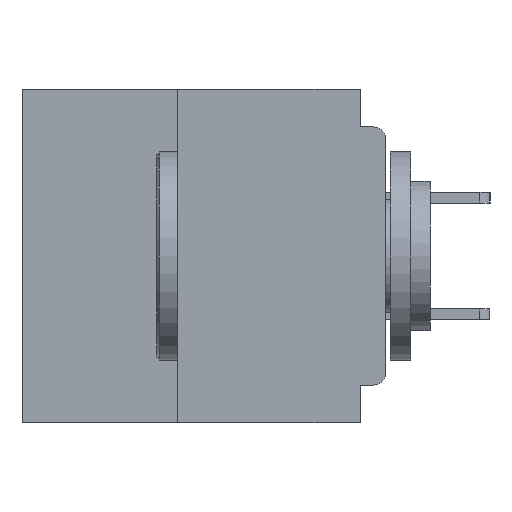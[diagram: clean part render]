
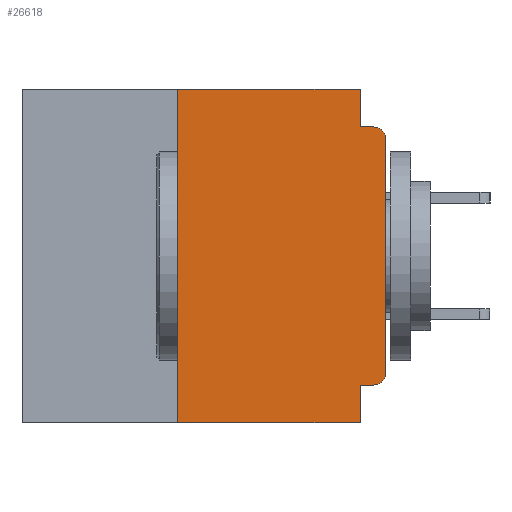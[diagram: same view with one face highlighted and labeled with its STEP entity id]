
A CAD part, left-side view. The second image highlights one B-rep face of the part: STEP entity #26618.
In plain terms, the highlighted planar face has unit normal (-1, 0, 0).
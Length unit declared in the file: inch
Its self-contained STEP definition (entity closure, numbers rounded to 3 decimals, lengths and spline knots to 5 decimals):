
#1320 = EDGE_CURVE ( 'NONE', #28242, #49609, #9044, .T. ) ;
#1909 = VERTEX_POINT ( 'NONE', #51159 ) ;
#2631 = DIRECTION ( 'NONE',  ( 0., 0., -1. ) ) ;
#3172 = ORIENTED_EDGE ( 'NONE', *, *, #53670, .T. ) ;
#4496 = DIRECTION ( 'NONE',  ( 0., 0., -1. ) ) ;
#6060 = VERTEX_POINT ( 'NONE', #48987 ) ;
#6602 = AXIS2_PLACEMENT_3D ( 'NONE', #45003, #19979, #49123 ) ;
#7800 = ORIENTED_EDGE ( 'NONE', *, *, #20304, .T. ) ;
#7839 = VECTOR ( 'NONE', #15477, 39.37008 ) ;
#7906 = LINE ( 'NONE', #22222, #30171 ) ;
#8903 = CARTESIAN_POINT ( 'NONE',  ( 0., 0.031, 0. ) ) ;
#9044 = LINE ( 'NONE', #44991, #41119 ) ;
#9107 = CARTESIAN_POINT ( 'NONE',  ( 0., 0., 0. ) ) ;
#10751 = LINE ( 'NONE', #48096, #52468 ) ;
#11008 = VECTOR ( 'NONE', #21540, 39.37008 ) ;
#12339 = CARTESIAN_POINT ( 'NONE',  ( 0., 0.437, -0.4 ) ) ;
#12829 = ORIENTED_EDGE ( 'NONE', *, *, #1320, .F. ) ;
#13657 = LINE ( 'NONE', #50643, #11008 ) ;
#14400 = ORIENTED_EDGE ( 'NONE', *, *, #47520, .T. ) ;
#15447 = VERTEX_POINT ( 'NONE', #40591 ) ;
#15477 = DIRECTION ( 'NONE',  ( 0., 0., 1. ) ) ;
#15708 = EDGE_CURVE ( 'NONE', #39594, #44630, #27010, .T. ) ;
#17530 = DIRECTION ( 'NONE',  ( 0., 0., 1. ) ) ;
#19979 = DIRECTION ( 'NONE',  ( -1., 0., 0. ) ) ;
#20304 = EDGE_CURVE ( 'NONE', #48693, #1909, #52551, .T. ) ;
#20799 = CIRCLE ( 'NONE', #35725, 0.015 ) ;
#21540 = DIRECTION ( 'NONE',  ( 0., -1., 0. ) ) ;
#21564 = LINE ( 'NONE', #9107, #42482 ) ;
#22110 = CARTESIAN_POINT ( 'NONE',  ( 0., 0.015, -0.355 ) ) ;
#22222 = CARTESIAN_POINT ( 'NONE',  ( 0., 0.437, 0. ) ) ;
#22454 = DIRECTION ( 'NONE',  ( -1., 0., 0. ) ) ;
#23320 = CARTESIAN_POINT ( 'NONE',  ( 0., 0.25, 0. ) ) ;
#23922 = CARTESIAN_POINT ( 'NONE',  ( 0., 0.25, -0.4 ) ) ;
#24081 = EDGE_CURVE ( 'NONE', #49609, #44619, #10751, .T. ) ;
#26618 = ADVANCED_FACE ( 'NONE', ( #28175 ), #44362, .F. ) ;
#27010 = LINE ( 'NONE', #8903, #46559 ) ;
#27082 = ORIENTED_EDGE ( 'NONE', *, *, #28877, .F. ) ;
#27754 = DIRECTION ( 'NONE',  ( 1., 0., 0. ) ) ;
#28175 = FACE_OUTER_BOUND ( 'NONE', #41848, .T. ) ;
#28242 = VERTEX_POINT ( 'NONE', #22110 ) ;
#28820 = CARTESIAN_POINT ( 'NONE',  ( 0., 0.031, -0.355 ) ) ;
#28877 = EDGE_CURVE ( 'NONE', #34270, #39594, #7906, .T. ) ;
#30171 = VECTOR ( 'NONE', #51311, 39.37008 ) ;
#31575 = VECTOR ( 'NONE', #45770, 39.37008 ) ;
#32268 = CARTESIAN_POINT ( 'NONE',  ( 0., 0.031, -0.045 ) ) ;
#32435 = AXIS2_PLACEMENT_3D ( 'NONE', #40168, #27754, #2631 ) ;
#32450 = CARTESIAN_POINT ( 'NONE',  ( 0., 0.031, -0.4 ) ) ;
#34270 = VERTEX_POINT ( 'NONE', #23320 ) ;
#35642 = EDGE_CURVE ( 'NONE', #15447, #34270, #52176, .T. ) ;
#35725 = AXIS2_PLACEMENT_3D ( 'NONE', #47407, #22454, #51539 ) ;
#36065 = EDGE_CURVE ( 'NONE', #6060, #48693, #21564, .T. ) ;
#36831 = ORIENTED_EDGE ( 'NONE', *, *, #41028, .F. ) ;
#37869 = ORIENTED_EDGE ( 'NONE', *, *, #36065, .T. ) ;
#39443 = ORIENTED_EDGE ( 'NONE', *, *, #24081, .F. ) ;
#39594 = VERTEX_POINT ( 'NONE', #45049 ) ;
#40168 = CARTESIAN_POINT ( 'NONE',  ( 0., 0.437, 0. ) ) ;
#40591 = CARTESIAN_POINT ( 'NONE',  ( 0., 0.25, -0.4 ) ) ;
#41028 = EDGE_CURVE ( 'NONE', #44630, #1909, #13657, .T. ) ;
#41119 = VECTOR ( 'NONE', #43690, 39.37008 ) ;
#41848 = EDGE_LOOP ( 'NONE', ( #37869, #7800, #36831, #48383, #27082, #43692, #3172, #39443, #12829, #14400 ) ) ;
#42482 = VECTOR ( 'NONE', #17530, 39.37008 ) ;
#42992 = CARTESIAN_POINT ( 'NONE',  ( 0., 0., -0.06 ) ) ;
#43690 = DIRECTION ( 'NONE',  ( 0., 1., 0. ) ) ;
#43692 = ORIENTED_EDGE ( 'NONE', *, *, #35642, .F. ) ;
#44027 = LINE ( 'NONE', #12339, #31575 ) ;
#44362 = PLANE ( 'NONE',  #32435 ) ;
#44619 = VERTEX_POINT ( 'NONE', #32450 ) ;
#44630 = VERTEX_POINT ( 'NONE', #32268 ) ;
#44991 = CARTESIAN_POINT ( 'NONE',  ( 0., 0., -0.355 ) ) ;
#45003 = CARTESIAN_POINT ( 'NONE',  ( 0., 0.015, -0.06 ) ) ;
#45049 = CARTESIAN_POINT ( 'NONE',  ( 0., 0.031, 0. ) ) ;
#45770 = DIRECTION ( 'NONE',  ( 0., -1., 0. ) ) ;
#46559 = VECTOR ( 'NONE', #4496, 39.37008 ) ;
#47407 = CARTESIAN_POINT ( 'NONE',  ( 0., 0.015, -0.34 ) ) ;
#47520 = EDGE_CURVE ( 'NONE', #28242, #6060, #20799, .T. ) ;
#48096 = CARTESIAN_POINT ( 'NONE',  ( 0., 0.031, -0.4 ) ) ;
#48271 = DIRECTION ( 'NONE',  ( 0., 0., -1. ) ) ;
#48383 = ORIENTED_EDGE ( 'NONE', *, *, #15708, .F. ) ;
#48693 = VERTEX_POINT ( 'NONE', #42992 ) ;
#48987 = CARTESIAN_POINT ( 'NONE',  ( 0., 0., -0.34 ) ) ;
#49123 = DIRECTION ( 'NONE',  ( 0., 0., -1. ) ) ;
#49609 = VERTEX_POINT ( 'NONE', #28820 ) ;
#50643 = CARTESIAN_POINT ( 'NONE',  ( 0., 0., -0.045 ) ) ;
#51159 = CARTESIAN_POINT ( 'NONE',  ( 0., 0.015, -0.045 ) ) ;
#51311 = DIRECTION ( 'NONE',  ( 0., -1., 0. ) ) ;
#51539 = DIRECTION ( 'NONE',  ( 0., 0., -1. ) ) ;
#52176 = LINE ( 'NONE', #23922, #7839 ) ;
#52468 = VECTOR ( 'NONE', #48271, 39.37008 ) ;
#52551 = CIRCLE ( 'NONE', #6602, 0.015 ) ;
#53670 = EDGE_CURVE ( 'NONE', #15447, #44619, #44027, .T. ) ;
